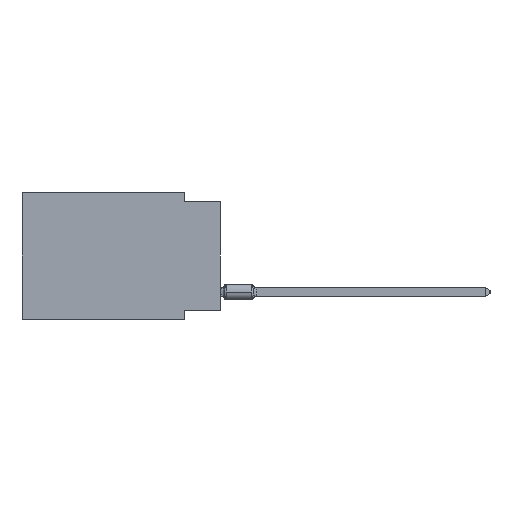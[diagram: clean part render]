
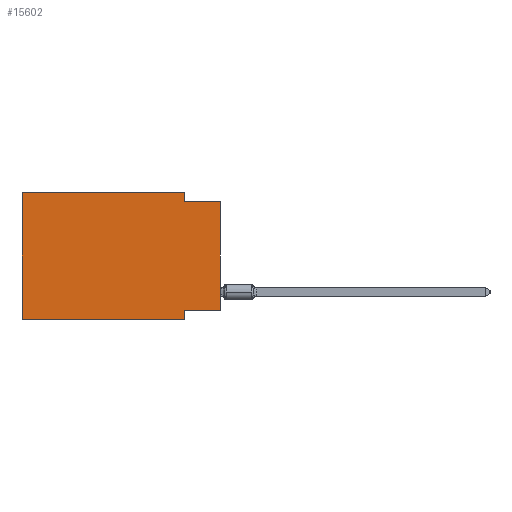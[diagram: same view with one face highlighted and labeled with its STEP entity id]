
A CAD part, left-side view. The second image highlights one B-rep face of the part: STEP entity #15602.
In plain terms, the highlighted planar face has unit normal (-1, 0, 0).
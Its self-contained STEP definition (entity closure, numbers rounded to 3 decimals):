
#34 = CARTESIAN_POINT ( 'NONE',  ( 0., 2.54, 0. ) ) ;
#182 = CARTESIAN_POINT ( 'NONE',  ( 0., 13.97, 0. ) ) ;
#1488 = AXIS2_PLACEMENT_3D ( 'NONE', #18431, #28303, #6950 ) ;
#1842 = VECTOR ( 'NONE', #16060, 1000. ) ;
#2085 = EDGE_CURVE ( 'NONE', #7395, #6455, #27652, .T. ) ;
#2348 = VECTOR ( 'NONE', #20723, 1000. ) ;
#2432 = VERTEX_POINT ( 'NONE', #30206 ) ;
#2714 = VERTEX_POINT ( 'NONE', #31663 ) ;
#2874 = EDGE_CURVE ( 'NONE', #27016, #2432, #21234, .T. ) ;
#3240 = DIRECTION ( 'NONE',  ( 0., 1., 0. ) ) ;
#3294 = ORIENTED_EDGE ( 'NONE', *, *, #23230, .T. ) ;
#4242 = CARTESIAN_POINT ( 'NONE',  ( 0., 0., 0. ) ) ;
#4571 = DIRECTION ( 'NONE',  ( 0., 0., 1. ) ) ;
#5071 = LINE ( 'NONE', #25419, #6587 ) ;
#6455 = VERTEX_POINT ( 'NONE', #23396 ) ;
#6587 = VECTOR ( 'NONE', #12968, 1000. ) ;
#6950 = DIRECTION ( 'NONE',  ( 0., 0., -1. ) ) ;
#7395 = VERTEX_POINT ( 'NONE', #23602 ) ;
#8088 = PLANE ( 'NONE',  #1488 ) ;
#8281 = CARTESIAN_POINT ( 'NONE',  ( 0., 13.97, 0. ) ) ;
#8360 = EDGE_CURVE ( 'NONE', #31958, #2714, #27171, .T. ) ;
#8373 = CARTESIAN_POINT ( 'NONE',  ( 0., 2.54, -0.635 ) ) ;
#9402 = EDGE_LOOP ( 'NONE', ( #3294, #22698, #16623, #20198, #20947, #19203, #30140, #31260 ) ) ;
#10041 = DIRECTION ( 'NONE',  ( 0., 0., 1. ) ) ;
#10635 = EDGE_CURVE ( 'NONE', #2714, #21788, #15398, .T. ) ;
#10903 = DIRECTION ( 'NONE',  ( 0., 0., -1. ) ) ;
#11805 = VECTOR ( 'NONE', #19594, 1000. ) ;
#12968 = DIRECTION ( 'NONE',  ( 0., 0., -1. ) ) ;
#13170 = LINE ( 'NONE', #20919, #23094 ) ;
#15398 = LINE ( 'NONE', #8281, #2348 ) ;
#15450 = EDGE_CURVE ( 'NONE', #31958, #30681, #30084, .T. ) ;
#15602 = ADVANCED_FACE ( 'NONE', ( #30738 ), #8088, .F. ) ;
#15831 = VECTOR ( 'NONE', #4571, 1000. ) ;
#15854 = CARTESIAN_POINT ( 'NONE',  ( 0., 0., -8.255 ) ) ;
#16060 = DIRECTION ( 'NONE',  ( 0., -1., 0. ) ) ;
#16623 = ORIENTED_EDGE ( 'NONE', *, *, #29334, .F. ) ;
#17288 = VECTOR ( 'NONE', #3240, 1000. ) ;
#17709 = CARTESIAN_POINT ( 'NONE',  ( 0., 13.97, -8.89 ) ) ;
#18431 = CARTESIAN_POINT ( 'NONE',  ( 0., 13.97, 0. ) ) ;
#19203 = ORIENTED_EDGE ( 'NONE', *, *, #15450, .T. ) ;
#19594 = DIRECTION ( 'NONE',  ( 0., -1., 0. ) ) ;
#20198 = ORIENTED_EDGE ( 'NONE', *, *, #10635, .F. ) ;
#20723 = DIRECTION ( 'NONE',  ( 0., -1., 0. ) ) ;
#20919 = CARTESIAN_POINT ( 'NONE',  ( 0., 2.54, -8.89 ) ) ;
#20947 = ORIENTED_EDGE ( 'NONE', *, *, #8360, .F. ) ;
#21234 = LINE ( 'NONE', #30957, #1842 ) ;
#21788 = VERTEX_POINT ( 'NONE', #34 ) ;
#22698 = ORIENTED_EDGE ( 'NONE', *, *, #2874, .F. ) ;
#22885 = VECTOR ( 'NONE', #10041, 1000. ) ;
#23048 = CARTESIAN_POINT ( 'NONE',  ( 0., 2.54, -8.89 ) ) ;
#23094 = VECTOR ( 'NONE', #10903, 1000. ) ;
#23230 = EDGE_CURVE ( 'NONE', #7395, #2432, #29290, .T. ) ;
#23396 = CARTESIAN_POINT ( 'NONE',  ( 0., 2.54, -8.255 ) ) ;
#23602 = CARTESIAN_POINT ( 'NONE',  ( 0., 0., -8.255 ) ) ;
#25419 = CARTESIAN_POINT ( 'NONE',  ( 0., 2.54, 0. ) ) ;
#27016 = VERTEX_POINT ( 'NONE', #8373 ) ;
#27171 = LINE ( 'NONE', #182, #22885 ) ;
#27652 = LINE ( 'NONE', #15854, #17288 ) ;
#28303 = DIRECTION ( 'NONE',  ( 1., 0., 0. ) ) ;
#29063 = EDGE_CURVE ( 'NONE', #6455, #30681, #13170, .T. ) ;
#29290 = LINE ( 'NONE', #4242, #15831 ) ;
#29334 = EDGE_CURVE ( 'NONE', #21788, #27016, #5071, .T. ) ;
#29612 = CARTESIAN_POINT ( 'NONE',  ( 0., 13.97, -8.89 ) ) ;
#30084 = LINE ( 'NONE', #29612, #11805 ) ;
#30140 = ORIENTED_EDGE ( 'NONE', *, *, #29063, .F. ) ;
#30206 = CARTESIAN_POINT ( 'NONE',  ( 0., 0., -0.635 ) ) ;
#30681 = VERTEX_POINT ( 'NONE', #23048 ) ;
#30738 = FACE_OUTER_BOUND ( 'NONE', #9402, .T. ) ;
#30957 = CARTESIAN_POINT ( 'NONE',  ( 0., 0., -0.635 ) ) ;
#31260 = ORIENTED_EDGE ( 'NONE', *, *, #2085, .F. ) ;
#31663 = CARTESIAN_POINT ( 'NONE',  ( 0., 13.97, 0. ) ) ;
#31958 = VERTEX_POINT ( 'NONE', #17709 ) ;
